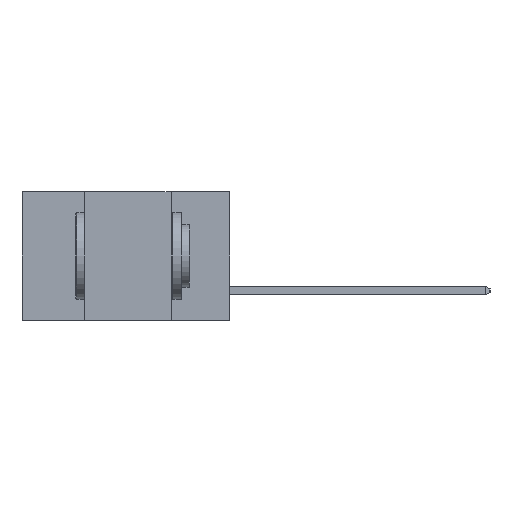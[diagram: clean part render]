
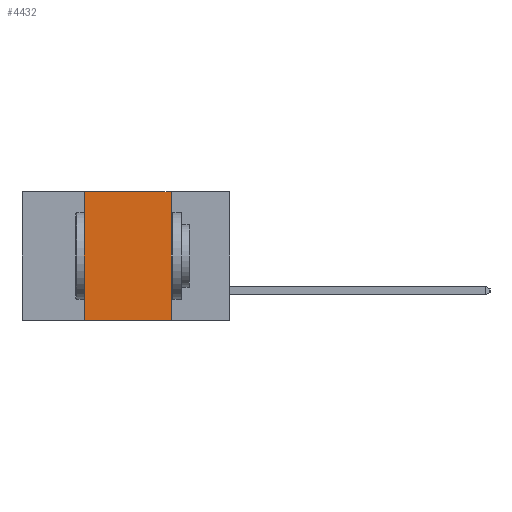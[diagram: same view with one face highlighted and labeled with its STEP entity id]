
A CAD part, left-side view. The second image highlights one B-rep face of the part: STEP entity #4432.
In plain terms, the highlighted planar face has unit normal (-1, 0, 0).
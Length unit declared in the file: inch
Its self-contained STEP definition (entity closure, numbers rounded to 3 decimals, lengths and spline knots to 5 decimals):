
#92 = AXIS2_PLACEMENT_3D ( 'NONE', #13057, #3025, #2976 ) ;
#1511 = FACE_OUTER_BOUND ( 'NONE', #2009, .T. ) ;
#1513 = VERTEX_POINT ( 'NONE', #11013 ) ;
#2009 = EDGE_LOOP ( 'NONE', ( #19252, #8892, #9542, #13101 ) ) ;
#2950 = DIRECTION ( 'NONE',  ( 0., 0., -1. ) ) ;
#2976 = DIRECTION ( 'NONE',  ( 0., 0., -1. ) ) ;
#3025 = DIRECTION ( 'NONE',  ( 1., 0., 0. ) ) ;
#3758 = PLANE ( 'NONE',  #92 ) ;
#3825 = LINE ( 'NONE', #18867, #13526 ) ;
#3878 = CARTESIAN_POINT ( 'NONE',  ( 0., 0.6, 0. ) ) ;
#4432 = ADVANCED_FACE ( 'NONE', ( #1511 ), #3758, .F. ) ;
#5201 = VERTEX_POINT ( 'NONE', #22284 ) ;
#6843 = LINE ( 'NONE', #17456, #15915 ) ;
#7844 = EDGE_CURVE ( 'NONE', #14899, #11472, #3825, .T. ) ;
#8765 = CARTESIAN_POINT ( 'NONE',  ( 0., 0.17, -0.37 ) ) ;
#8892 = ORIENTED_EDGE ( 'NONE', *, *, #14716, .F. ) ;
#9542 = ORIENTED_EDGE ( 'NONE', *, *, #12685, .F. ) ;
#10227 = LINE ( 'NONE', #21513, #14447 ) ;
#11013 = CARTESIAN_POINT ( 'NONE',  ( 0., 0.42, 0. ) ) ;
#11472 = VERTEX_POINT ( 'NONE', #8765 ) ;
#12685 = EDGE_CURVE ( 'NONE', #14899, #1513, #10227, .T. ) ;
#13057 = CARTESIAN_POINT ( 'NONE',  ( 0., 0.6, 0. ) ) ;
#13101 = ORIENTED_EDGE ( 'NONE', *, *, #7844, .T. ) ;
#13526 = VECTOR ( 'NONE', #18989, 39.37008 ) ;
#14447 = VECTOR ( 'NONE', #23198, 39.37008 ) ;
#14716 = EDGE_CURVE ( 'NONE', #1513, #5201, #18531, .T. ) ;
#14899 = VERTEX_POINT ( 'NONE', #22314 ) ;
#15915 = VECTOR ( 'NONE', #2950, 39.37008 ) ;
#16639 = DIRECTION ( 'NONE',  ( 0., -1., 0. ) ) ;
#17456 = CARTESIAN_POINT ( 'NONE',  ( 0., 0.17, 0. ) ) ;
#18531 = LINE ( 'NONE', #3878, #23169 ) ;
#18867 = CARTESIAN_POINT ( 'NONE',  ( 0., 0.6, -0.37 ) ) ;
#18989 = DIRECTION ( 'NONE',  ( 0., -1., 0. ) ) ;
#19252 = ORIENTED_EDGE ( 'NONE', *, *, #20024, .F. ) ;
#20024 = EDGE_CURVE ( 'NONE', #5201, #11472, #6843, .T. ) ;
#21513 = CARTESIAN_POINT ( 'NONE',  ( 0., 0.42, 0. ) ) ;
#22284 = CARTESIAN_POINT ( 'NONE',  ( 0., 0.17, 0. ) ) ;
#22314 = CARTESIAN_POINT ( 'NONE',  ( 0., 0.42, -0.37 ) ) ;
#23169 = VECTOR ( 'NONE', #16639, 39.37008 ) ;
#23198 = DIRECTION ( 'NONE',  ( 0., 0., 1. ) ) ;
